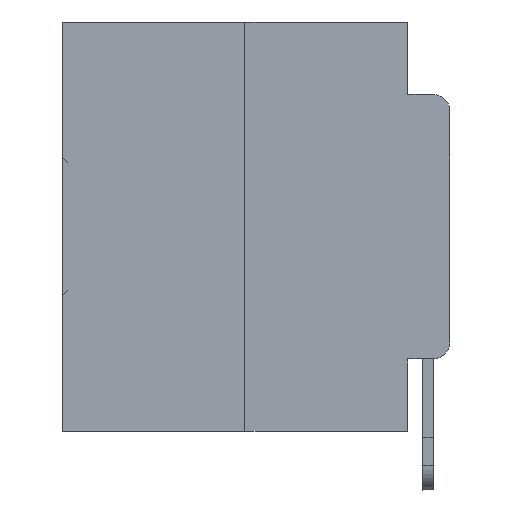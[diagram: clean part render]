
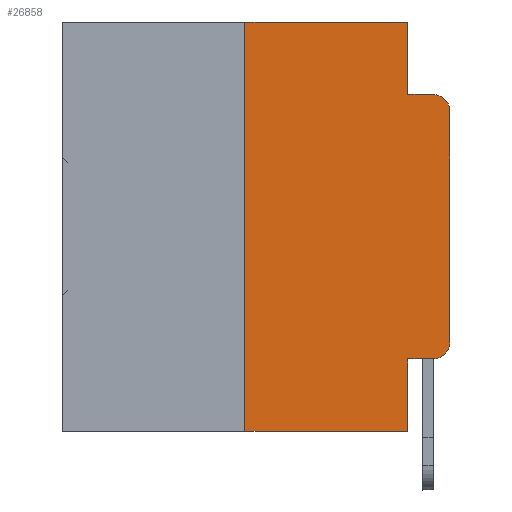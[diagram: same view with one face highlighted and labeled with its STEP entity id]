
A CAD part, left-side view. The second image highlights one B-rep face of the part: STEP entity #26858.
In plain terms, the highlighted planar face has unit normal (-1, 0, 0).
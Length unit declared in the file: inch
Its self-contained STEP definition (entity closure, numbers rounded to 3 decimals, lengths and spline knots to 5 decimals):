
#701 = LINE ( 'NONE', #15324, #14330 ) ;
#1369 = CARTESIAN_POINT ( 'NONE',  ( 0., 0.02, -0.3915 ) ) ;
#1455 = CIRCLE ( 'NONE', #10671, 0.02 ) ;
#1639 = DIRECTION ( 'NONE',  ( 0., -1., 0. ) ) ;
#1767 = EDGE_CURVE ( 'NONE', #32290, #4679, #4668, .T. ) ;
#1983 = EDGE_LOOP ( 'NONE', ( #28932, #10075, #13718, #5349, #28856, #27017, #19987, #28495, #10186, #16305 ) ) ;
#2105 = EDGE_CURVE ( 'NONE', #20517, #17684, #14441, .T. ) ;
#2145 = FACE_OUTER_BOUND ( 'NONE', #1983, .T. ) ;
#3268 = EDGE_CURVE ( 'NONE', #4925, #8078, #12126, .T. ) ;
#3629 = PLANE ( 'NONE',  #35156 ) ;
#4668 = LINE ( 'NONE', #22417, #33941 ) ;
#4679 = VERTEX_POINT ( 'NONE', #29363 ) ;
#4925 = VERTEX_POINT ( 'NONE', #6353 ) ;
#4996 = CARTESIAN_POINT ( 'NONE',  ( 0., 0.051, -0.5 ) ) ;
#5349 = ORIENTED_EDGE ( 'NONE', *, *, #27962, .F. ) ;
#5805 = DIRECTION ( 'NONE',  ( 0., -1., 0. ) ) ;
#5896 = LINE ( 'NONE', #16053, #13290 ) ;
#6059 = DIRECTION ( 'NONE',  ( 0., 0., -1. ) ) ;
#6244 = CARTESIAN_POINT ( 'NONE',  ( 0., 0.473, 0. ) ) ;
#6353 = CARTESIAN_POINT ( 'NONE',  ( 0., 0.051, -0.0885 ) ) ;
#6384 = VECTOR ( 'NONE', #18155, 39.37008 ) ;
#6765 = EDGE_CURVE ( 'NONE', #13690, #8078, #30066, .T. ) ;
#7168 = CARTESIAN_POINT ( 'NONE',  ( 0., 0.473, -0.5 ) ) ;
#8078 = VERTEX_POINT ( 'NONE', #30263 ) ;
#8977 = VERTEX_POINT ( 'NONE', #14929 ) ;
#9011 = DIRECTION ( 'NONE',  ( 0., 0., -1. ) ) ;
#9434 = EDGE_CURVE ( 'NONE', #8977, #29077, #1455, .T. ) ;
#9448 = DIRECTION ( 'NONE',  ( 1., 0., 0. ) ) ;
#10075 = ORIENTED_EDGE ( 'NONE', *, *, #6765, .T. ) ;
#10186 = ORIENTED_EDGE ( 'NONE', *, *, #11763, .T. ) ;
#10671 = AXIS2_PLACEMENT_3D ( 'NONE', #1369, #34127, #22688 ) ;
#11683 = CARTESIAN_POINT ( 'NONE',  ( 0., 0., 0. ) ) ;
#11763 = EDGE_CURVE ( 'NONE', #20517, #8977, #701, .T. ) ;
#11803 = DIRECTION ( 'NONE',  ( 0., 0., 1. ) ) ;
#12126 = LINE ( 'NONE', #12781, #32898 ) ;
#12179 = DIRECTION ( 'NONE',  ( 0., 0., -1. ) ) ;
#12461 = AXIS2_PLACEMENT_3D ( 'NONE', #31021, #30901, #23037 ) ;
#12781 = CARTESIAN_POINT ( 'NONE',  ( 0., 0.051, -0.0885 ) ) ;
#13290 = VECTOR ( 'NONE', #24921, 39.37008 ) ;
#13674 = CARTESIAN_POINT ( 'NONE',  ( 0., 0., -0.1085 ) ) ;
#13690 = VERTEX_POINT ( 'NONE', #13674 ) ;
#13718 = ORIENTED_EDGE ( 'NONE', *, *, #3268, .F. ) ;
#14080 = VECTOR ( 'NONE', #11803, 39.37008 ) ;
#14330 = VECTOR ( 'NONE', #5805, 39.37008 ) ;
#14372 = CARTESIAN_POINT ( 'NONE',  ( 0., 0.051, 0. ) ) ;
#14441 = LINE ( 'NONE', #14372, #21164 ) ;
#14929 = CARTESIAN_POINT ( 'NONE',  ( 0., 0.02, -0.4115 ) ) ;
#15324 = CARTESIAN_POINT ( 'NONE',  ( 0., 0.051, -0.4115 ) ) ;
#16053 = CARTESIAN_POINT ( 'NONE',  ( 0., 0.473, 0. ) ) ;
#16305 = ORIENTED_EDGE ( 'NONE', *, *, #9434, .T. ) ;
#16686 = VERTEX_POINT ( 'NONE', #30402 ) ;
#17684 = VERTEX_POINT ( 'NONE', #4996 ) ;
#18155 = DIRECTION ( 'NONE',  ( 0., -1., 0. ) ) ;
#18628 = CARTESIAN_POINT ( 'NONE',  ( 0., 0., -0.3915 ) ) ;
#19987 = ORIENTED_EDGE ( 'NONE', *, *, #27688, .T. ) ;
#20517 = VERTEX_POINT ( 'NONE', #31805 ) ;
#21164 = VECTOR ( 'NONE', #6059, 39.37008 ) ;
#21601 = LINE ( 'NONE', #7168, #6384 ) ;
#22417 = CARTESIAN_POINT ( 'NONE',  ( 0., 0.25, 0. ) ) ;
#22540 = DIRECTION ( 'NONE',  ( 0., 0., 1. ) ) ;
#22688 = DIRECTION ( 'NONE',  ( 0., 0., -1. ) ) ;
#23037 = DIRECTION ( 'NONE',  ( 0., 0., -1. ) ) ;
#24195 = EDGE_CURVE ( 'NONE', #4679, #16686, #5896, .T. ) ;
#24568 = LINE ( 'NONE', #33227, #30529 ) ;
#24653 = LINE ( 'NONE', #11683, #14080 ) ;
#24921 = DIRECTION ( 'NONE',  ( 0., -1., 0. ) ) ;
#26107 = EDGE_CURVE ( 'NONE', #29077, #13690, #24653, .T. ) ;
#26858 = ADVANCED_FACE ( 'NONE', ( #2145 ), #3629, .F. ) ;
#27017 = ORIENTED_EDGE ( 'NONE', *, *, #1767, .F. ) ;
#27688 = EDGE_CURVE ( 'NONE', #32290, #17684, #21601, .T. ) ;
#27962 = EDGE_CURVE ( 'NONE', #16686, #4925, #24568, .T. ) ;
#28495 = ORIENTED_EDGE ( 'NONE', *, *, #2105, .F. ) ;
#28856 = ORIENTED_EDGE ( 'NONE', *, *, #24195, .F. ) ;
#28932 = ORIENTED_EDGE ( 'NONE', *, *, #26107, .T. ) ;
#29077 = VERTEX_POINT ( 'NONE', #18628 ) ;
#29363 = CARTESIAN_POINT ( 'NONE',  ( 0., 0.25, 0. ) ) ;
#30066 = CIRCLE ( 'NONE', #12461, 0.02 ) ;
#30263 = CARTESIAN_POINT ( 'NONE',  ( 0., 0.02, -0.0885 ) ) ;
#30402 = CARTESIAN_POINT ( 'NONE',  ( 0., 0.051, 0. ) ) ;
#30529 = VECTOR ( 'NONE', #9011, 39.37008 ) ;
#30812 = CARTESIAN_POINT ( 'NONE',  ( 0., 0.25, -0.5 ) ) ;
#30901 = DIRECTION ( 'NONE',  ( -1., 0., 0. ) ) ;
#31021 = CARTESIAN_POINT ( 'NONE',  ( 0., 0.02, -0.1085 ) ) ;
#31805 = CARTESIAN_POINT ( 'NONE',  ( 0., 0.051, -0.4115 ) ) ;
#32290 = VERTEX_POINT ( 'NONE', #30812 ) ;
#32898 = VECTOR ( 'NONE', #1639, 39.37008 ) ;
#33227 = CARTESIAN_POINT ( 'NONE',  ( 0., 0.051, 0. ) ) ;
#33941 = VECTOR ( 'NONE', #22540, 39.37008 ) ;
#34127 = DIRECTION ( 'NONE',  ( -1., 0., 0. ) ) ;
#35156 = AXIS2_PLACEMENT_3D ( 'NONE', #6244, #9448, #12179 ) ;
